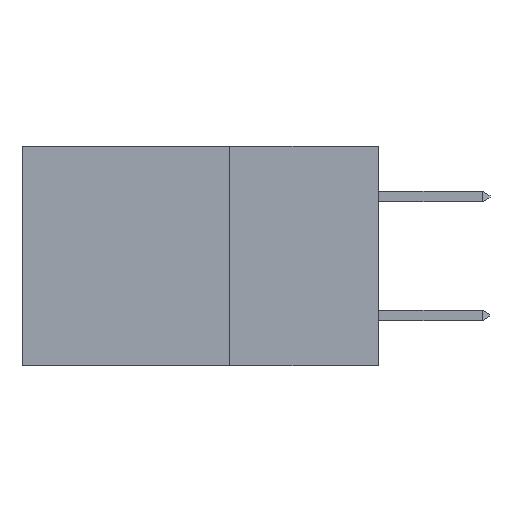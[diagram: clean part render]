
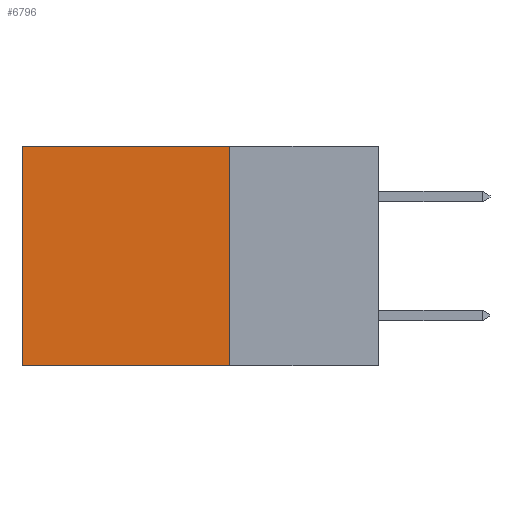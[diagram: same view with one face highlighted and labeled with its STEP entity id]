
A CAD part, left-side view. The second image highlights one B-rep face of the part: STEP entity #6796.
In plain terms, the highlighted planar face has unit normal (-1, 0, 0).
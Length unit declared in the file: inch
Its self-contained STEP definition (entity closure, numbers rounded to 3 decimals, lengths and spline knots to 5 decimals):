
#412 = VERTEX_POINT ( 'NONE', #614 ) ;
#488 = ORIENTED_EDGE ( 'NONE', *, *, #15763, .F. ) ;
#614 = CARTESIAN_POINT ( 'NONE',  ( 0.298, 0.6, -0.37 ) ) ;
#857 = ORIENTED_EDGE ( 'NONE', *, *, #9486, .F. ) ;
#1609 = VERTEX_POINT ( 'NONE', #3109 ) ;
#1620 = ORIENTED_EDGE ( 'NONE', *, *, #12744, .T. ) ;
#1913 = CARTESIAN_POINT ( 'NONE',  ( 0.298, 0.25, 0. ) ) ;
#2023 = EDGE_CURVE ( 'NONE', #1609, #412, #6480, .T. ) ;
#2612 = DIRECTION ( 'NONE',  ( 0., 1., 0. ) ) ;
#3109 = CARTESIAN_POINT ( 'NONE',  ( 0.298, 0.6, 0. ) ) ;
#4009 = CARTESIAN_POINT ( 'NONE',  ( 0.298, 0.25, -0.37 ) ) ;
#4591 = CARTESIAN_POINT ( 'NONE',  ( 0.298, 0.25, -0.37 ) ) ;
#5066 = CARTESIAN_POINT ( 'NONE',  ( 0.298, 0.25, 0. ) ) ;
#5594 = DIRECTION ( 'NONE',  ( 0., 0., -1. ) ) ;
#6457 = DIRECTION ( 'NONE',  ( 0., 0., -1. ) ) ;
#6480 = LINE ( 'NONE', #7865, #16001 ) ;
#6796 = ADVANCED_FACE ( 'NONE', ( #7443 ), #11919, .F. ) ;
#7443 = FACE_OUTER_BOUND ( 'NONE', #10404, .T. ) ;
#7657 = ORIENTED_EDGE ( 'NONE', *, *, #2023, .T. ) ;
#7865 = CARTESIAN_POINT ( 'NONE',  ( 0.298, 0.6, 0. ) ) ;
#8164 = CARTESIAN_POINT ( 'NONE',  ( 0.298, 0.25, 0. ) ) ;
#8253 = LINE ( 'NONE', #10486, #11869 ) ;
#9486 = EDGE_CURVE ( 'NONE', #17801, #12762, #8253, .T. ) ;
#10404 = EDGE_LOOP ( 'NONE', ( #7657, #488, #857, #1620 ) ) ;
#10486 = CARTESIAN_POINT ( 'NONE',  ( 0.298, 0.25, 0. ) ) ;
#11834 = DIRECTION ( 'NONE',  ( 0., 0., -1. ) ) ;
#11869 = VECTOR ( 'NONE', #11834, 39.37008 ) ;
#11919 = PLANE ( 'NONE',  #12169 ) ;
#11949 = VECTOR ( 'NONE', #2612, 39.37008 ) ;
#12169 = AXIS2_PLACEMENT_3D ( 'NONE', #5066, #14579, #6457 ) ;
#12744 = EDGE_CURVE ( 'NONE', #17801, #1609, #15469, .T. ) ;
#12762 = VERTEX_POINT ( 'NONE', #4009 ) ;
#14579 = DIRECTION ( 'NONE',  ( 1., 0., 0. ) ) ;
#15257 = VECTOR ( 'NONE', #15459, 39.37008 ) ;
#15459 = DIRECTION ( 'NONE',  ( 0., 1., 0. ) ) ;
#15469 = LINE ( 'NONE', #8164, #11949 ) ;
#15670 = LINE ( 'NONE', #4591, #15257 ) ;
#15763 = EDGE_CURVE ( 'NONE', #12762, #412, #15670, .T. ) ;
#16001 = VECTOR ( 'NONE', #5594, 39.37008 ) ;
#17801 = VERTEX_POINT ( 'NONE', #1913 ) ;
